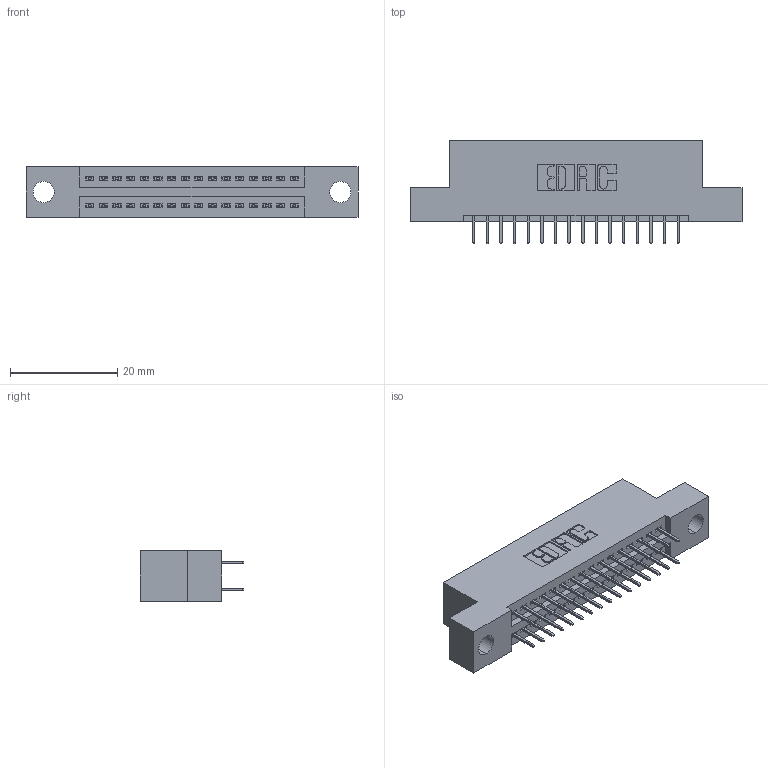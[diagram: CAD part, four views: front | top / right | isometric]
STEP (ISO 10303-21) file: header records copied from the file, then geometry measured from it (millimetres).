
FILE_DESCRIPTION (( 'STEP AP203' ), '1' );
FILE_NAME ('395-032-524-204.STEP', '2021-06-16T20:25:03', ( '' ), ( '' ), 'SwSTEP 2.0', 'SolidWorks 2020', '' );
FILE_SCHEMA (( 'CONFIG_CONTROL_DESIGN' ));
Length unit declared in the file: inch
Products named in the file (3): 345 Part_Flush Mounting Lugs - 0.156 Dia-TI; 395-032-524-204; 345-292-001_345-293-124
Assembly tree (33 placements, depth 2):
  395-032-524-204
    345 Part_Flush Mounting Lugs - 0.156 Dia-TI
    345-292-001_345-293-124  x32
Bounding box: 61.85 x 19.35 x 9.4 mm (x, y, z)
Volume: 5612.4 mm3; surface area: 7516.2 mm2
Topology: 33 solids, 33 shells, 1868 faces, 5273 edges, 3386 vertices
Faces by surface type: plane 1342, cylinder 526
Entity records: 16547 total; most frequent: CARTESIAN_POINT 2802, ORIENTED_EDGE 2734, DIRECTION 2503, EDGE_CURVE 1367, VECTOR 1175, LINE 1175, VERTEX_POINT 906, AXIS2_PLACEMENT_3D 664
